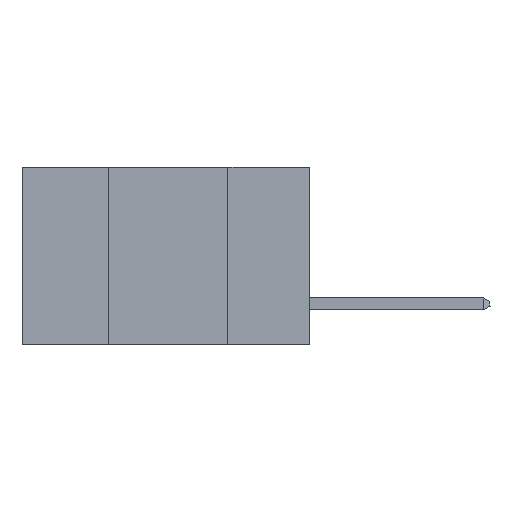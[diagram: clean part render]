
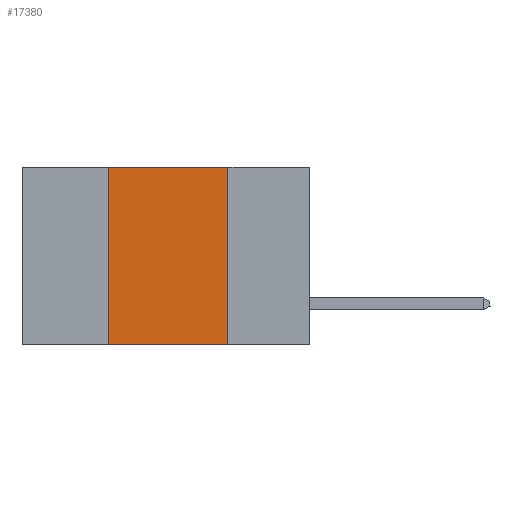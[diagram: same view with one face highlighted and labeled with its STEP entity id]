
A CAD part, left-side view. The second image highlights one B-rep face of the part: STEP entity #17380.
In plain terms, the highlighted planar face has unit normal (-1, 0, 0).
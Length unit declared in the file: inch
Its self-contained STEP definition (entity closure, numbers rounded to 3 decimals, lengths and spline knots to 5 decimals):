
#654 = CARTESIAN_POINT ( 'NONE',  ( 0., 0.17, 0. ) ) ;
#1069 = EDGE_CURVE ( 'NONE', #10694, #7962, #9687, .T. ) ;
#1690 = EDGE_LOOP ( 'NONE', ( #10015, #12769, #6521, #3245 ) ) ;
#2142 = DIRECTION ( 'NONE',  ( 0., -1., 0. ) ) ;
#3245 = ORIENTED_EDGE ( 'NONE', *, *, #1069, .T. ) ;
#3870 = CARTESIAN_POINT ( 'NONE',  ( 0., 0.42, 0. ) ) ;
#4054 = VECTOR ( 'NONE', #2142, 39.37008 ) ;
#4136 = CARTESIAN_POINT ( 'NONE',  ( 0., 0.6, 0. ) ) ;
#4978 = AXIS2_PLACEMENT_3D ( 'NONE', #4136, #5545, #17264 ) ;
#5222 = CARTESIAN_POINT ( 'NONE',  ( 0., 0.17, 0. ) ) ;
#5545 = DIRECTION ( 'NONE',  ( 1., 0., 0. ) ) ;
#5805 = CARTESIAN_POINT ( 'NONE',  ( 0., 0.6, 0. ) ) ;
#5816 = VECTOR ( 'NONE', #18202, 39.37008 ) ;
#6521 = ORIENTED_EDGE ( 'NONE', *, *, #10569, .F. ) ;
#6619 = CARTESIAN_POINT ( 'NONE',  ( 0., 0.6, -0.37 ) ) ;
#7962 = VERTEX_POINT ( 'NONE', #16106 ) ;
#9405 = FACE_OUTER_BOUND ( 'NONE', #1690, .T. ) ;
#9687 = LINE ( 'NONE', #6619, #14041 ) ;
#9917 = LINE ( 'NONE', #654, #5816 ) ;
#10015 = ORIENTED_EDGE ( 'NONE', *, *, #15194, .F. ) ;
#10204 = VERTEX_POINT ( 'NONE', #5222 ) ;
#10569 = EDGE_CURVE ( 'NONE', #10694, #13267, #12673, .T. ) ;
#10694 = VERTEX_POINT ( 'NONE', #16245 ) ;
#11473 = PLANE ( 'NONE',  #4978 ) ;
#12673 = LINE ( 'NONE', #18027, #18583 ) ;
#12769 = ORIENTED_EDGE ( 'NONE', *, *, #16218, .F. ) ;
#13267 = VERTEX_POINT ( 'NONE', #3870 ) ;
#13965 = DIRECTION ( 'NONE',  ( 0., -1., 0. ) ) ;
#14041 = VECTOR ( 'NONE', #13965, 39.37008 ) ;
#14335 = DIRECTION ( 'NONE',  ( 0., 0., 1. ) ) ;
#15194 = EDGE_CURVE ( 'NONE', #10204, #7962, #9917, .T. ) ;
#16106 = CARTESIAN_POINT ( 'NONE',  ( 0., 0.17, -0.37 ) ) ;
#16218 = EDGE_CURVE ( 'NONE', #13267, #10204, #17429, .T. ) ;
#16245 = CARTESIAN_POINT ( 'NONE',  ( 0., 0.42, -0.37 ) ) ;
#17264 = DIRECTION ( 'NONE',  ( 0., 0., -1. ) ) ;
#17380 = ADVANCED_FACE ( 'NONE', ( #9405 ), #11473, .F. ) ;
#17429 = LINE ( 'NONE', #5805, #4054 ) ;
#18027 = CARTESIAN_POINT ( 'NONE',  ( 0., 0.42, 0. ) ) ;
#18202 = DIRECTION ( 'NONE',  ( 0., 0., -1. ) ) ;
#18583 = VECTOR ( 'NONE', #14335, 39.37008 ) ;
